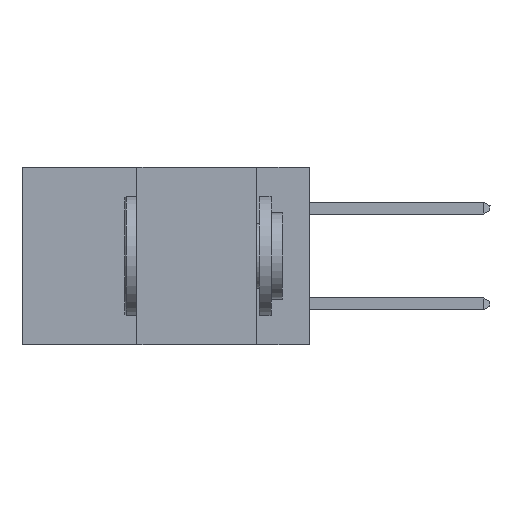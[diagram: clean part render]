
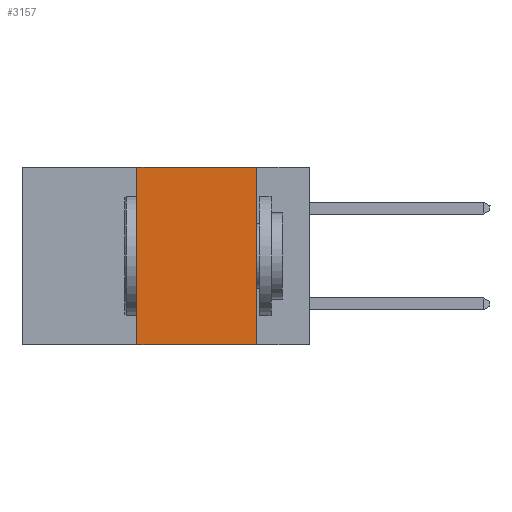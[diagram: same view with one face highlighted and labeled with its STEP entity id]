
A CAD part, left-side view. The second image highlights one B-rep face of the part: STEP entity #3157.
In plain terms, the highlighted planar face has unit normal (-1, 0, 0).
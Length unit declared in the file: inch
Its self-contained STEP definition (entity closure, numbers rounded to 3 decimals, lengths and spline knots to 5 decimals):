
#493 = CARTESIAN_POINT ( 'NONE',  ( 0., 0.36, 0. ) ) ;
#2092 = ORIENTED_EDGE ( 'NONE', *, *, #23228, .T. ) ;
#3021 = EDGE_CURVE ( 'NONE', #11997, #28375, #14533, .T. ) ;
#3157 = ADVANCED_FACE ( 'NONE', ( #8895 ), #13963, .F. ) ;
#3687 = CARTESIAN_POINT ( 'NONE',  ( 0., 0.36, -0.37 ) ) ;
#5334 = CARTESIAN_POINT ( 'NONE',  ( 0., 0.11, -0.37 ) ) ;
#5712 = EDGE_LOOP ( 'NONE', ( #13694, #19745, #34520, #2092 ) ) ;
#5953 = CARTESIAN_POINT ( 'NONE',  ( 0., 0.11, 0. ) ) ;
#7564 = VECTOR ( 'NONE', #23327, 39.37008 ) ;
#8895 = FACE_OUTER_BOUND ( 'NONE', #5712, .T. ) ;
#10403 = CARTESIAN_POINT ( 'NONE',  ( 0., 0.6, 0. ) ) ;
#11997 = VERTEX_POINT ( 'NONE', #5953 ) ;
#13694 = ORIENTED_EDGE ( 'NONE', *, *, #3021, .F. ) ;
#13963 = PLANE ( 'NONE',  #24381 ) ;
#14108 = CARTESIAN_POINT ( 'NONE',  ( 0., 0.6, 0. ) ) ;
#14533 = LINE ( 'NONE', #29479, #23747 ) ;
#16102 = DIRECTION ( 'NONE',  ( 0., 0., -1. ) ) ;
#16237 = LINE ( 'NONE', #493, #7564 ) ;
#17564 = CARTESIAN_POINT ( 'NONE',  ( 0., 0.36, 0. ) ) ;
#18548 = VERTEX_POINT ( 'NONE', #3687 ) ;
#19745 = ORIENTED_EDGE ( 'NONE', *, *, #41140, .F. ) ;
#21989 = EDGE_CURVE ( 'NONE', #18548, #33220, #16237, .T. ) ;
#23228 = EDGE_CURVE ( 'NONE', #18548, #28375, #26890, .T. ) ;
#23249 = DIRECTION ( 'NONE',  ( 0., 0., -1. ) ) ;
#23327 = DIRECTION ( 'NONE',  ( 0., 0., 1. ) ) ;
#23747 = VECTOR ( 'NONE', #16102, 39.37008 ) ;
#24381 = AXIS2_PLACEMENT_3D ( 'NONE', #14108, #36884, #23249 ) ;
#25496 = LINE ( 'NONE', #10403, #36122 ) ;
#26890 = LINE ( 'NONE', #38135, #31952 ) ;
#28375 = VERTEX_POINT ( 'NONE', #5334 ) ;
#29479 = CARTESIAN_POINT ( 'NONE',  ( 0., 0.11, 0. ) ) ;
#31952 = VECTOR ( 'NONE', #32152, 39.37008 ) ;
#32152 = DIRECTION ( 'NONE',  ( 0., -1., 0. ) ) ;
#32673 = DIRECTION ( 'NONE',  ( 0., -1., 0. ) ) ;
#33220 = VERTEX_POINT ( 'NONE', #17564 ) ;
#34520 = ORIENTED_EDGE ( 'NONE', *, *, #21989, .F. ) ;
#36122 = VECTOR ( 'NONE', #32673, 39.37008 ) ;
#36884 = DIRECTION ( 'NONE',  ( 1., 0., 0. ) ) ;
#38135 = CARTESIAN_POINT ( 'NONE',  ( 0., 0.6, -0.37 ) ) ;
#41140 = EDGE_CURVE ( 'NONE', #33220, #11997, #25496, .T. ) ;
